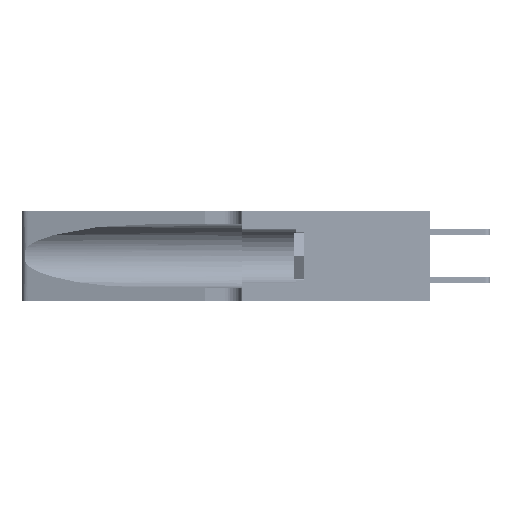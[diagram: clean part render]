
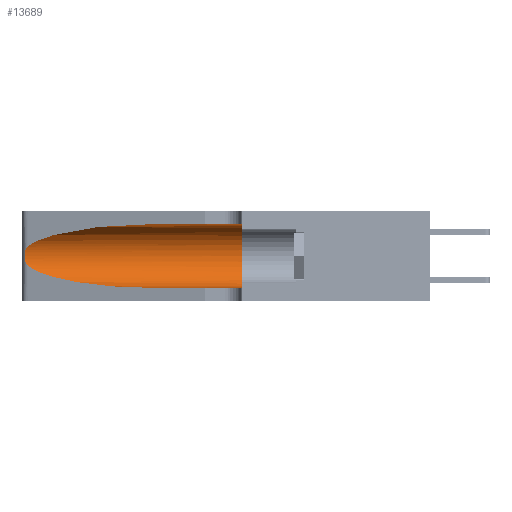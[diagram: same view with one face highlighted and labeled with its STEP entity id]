
A CAD part, left-side view. The second image highlights one B-rep face of the part: STEP entity #13689.
In plain terms, the highlighted cylindrical face has radius 3.308 mm (diameter 6.617 mm), a partial arc.
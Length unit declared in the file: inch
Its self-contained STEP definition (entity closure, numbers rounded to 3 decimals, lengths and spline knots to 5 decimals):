
#970 = CARTESIAN_POINT ( 'NONE',  ( 0.25487, 1.22718, 0.22369 ) ) ;
#1554 = CARTESIAN_POINT ( 'NONE',  ( 0.26075, 1.23896, 0.19203 ) ) ;
#2372 = CARTESIAN_POINT ( 'NONE',  ( 0.25856, 1.23593, 0.16098 ) ) ;
#3456 = CARTESIAN_POINT ( 'NONE',  ( 0.25487, 1.22718, 0.14631 ) ) ;
#3938 = CARTESIAN_POINT ( 'NONE',  ( 0.25487, 1.22718, 0.22369 ) ) ;
#5405 = ORIENTED_EDGE ( 'NONE', *, *, #24044, .T. ) ;
#6078 = EDGE_CURVE ( 'NONE', #14288, #38441, #24843, .T. ) ;
#6222 = EDGE_CURVE ( 'NONE', #24188, #38441, #10200, .T. ) ;
#6293 = VECTOR ( 'NONE', #38115, 39.37008 ) ;
#6353 = ORIENTED_EDGE ( 'NONE', *, *, #6222, .F. ) ;
#7549 = CARTESIAN_POINT ( 'NONE',  ( 0.1305, 0.72297, 0.31525 ) ) ;
#8357 = CARTESIAN_POINT ( 'NONE',  ( 0.1305, 0.35, 0.05475 ) ) ;
#8794 =( BOUNDED_CURVE ( )  B_SPLINE_CURVE ( 3, ( #12885, #34655, #16404, #22267 ),
 .UNSPECIFIED., .F., .F. ) 
 B_SPLINE_CURVE_WITH_KNOTS ( ( 4, 4 ),
 ( 3.44316, 4.71239 ),
 .UNSPECIFIED. ) 
 CURVE ( )  GEOMETRIC_REPRESENTATION_ITEM ( )  RATIONAL_B_SPLINE_CURVE ( ( 1., 0.87, 0.87, 1. ) ) 
 REPRESENTATION_ITEM ( '' )  );
#9586 = FACE_OUTER_BOUND ( 'NONE', #21133, .T. ) ;
#9924 = EDGE_CURVE ( 'NONE', #34025, #24188, #18055, .T. ) ;
#10067 = ORIENTED_EDGE ( 'NONE', *, *, #10087, .T. ) ;
#10087 = EDGE_CURVE ( 'NONE', #34557, #23011, #29959, .T. ) ;
#10200 = CIRCLE ( 'NONE', #36491, 0.13025 ) ;
#11184 = CARTESIAN_POINT ( 'NONE',  ( 0.2373, 1.15595, 0.28018 ) ) ;
#11263 = CARTESIAN_POINT ( 'NONE',  ( 0.25787, 1.23484, 0.2124 ) ) ;
#11590 = CARTESIAN_POINT ( 'NONE',  ( 0.25487, 1.22718, 0.22369 ) ) ;
#12116 = CARTESIAN_POINT ( 'NONE',  ( 0.1305, 0.35, 0.31525 ) ) ;
#12885 = CARTESIAN_POINT ( 'NONE',  ( 0.25487, 1.22718, 0.14631 ) ) ;
#12967 = ORIENTED_EDGE ( 'NONE', *, *, #6078, .T. ) ;
#13513 = CYLINDRICAL_SURFACE ( 'NONE', #17879, 0.13025 ) ;
#13689 = ADVANCED_FACE ( 'NONE', ( #9586 ), #13513, .F. ) ;
#14288 = VERTEX_POINT ( 'NONE', #37192 ) ;
#15039 = CARTESIAN_POINT ( 'NONE',  ( 0.26017, 1.23833, 0.17102 ) ) ;
#15421 = DIRECTION ( 'NONE',  ( 0., -1., 0. ) ) ;
#16009 = EDGE_CURVE ( 'NONE', #23011, #14288, #8794, .T. ) ;
#16404 = CARTESIAN_POINT ( 'NONE',  ( 0.18966, 0.96281, 0.05475 ) ) ;
#16839 = CARTESIAN_POINT ( 'NONE',  ( 0.25555, 1.22994, 0.2215 ) ) ;
#17711 = CARTESIAN_POINT ( 'NONE',  ( 0.18966, 0.96281, 0.31525 ) ) ;
#17795 = CARTESIAN_POINT ( 'NONE',  ( 0.26075, 1.23896, 0.178 ) ) ;
#17811 =( BOUNDED_CURVE ( )  B_SPLINE_CURVE ( 3, ( #36638, #17711, #11184, #11590 ),
 .UNSPECIFIED., .F., .F. ) 
 B_SPLINE_CURVE_WITH_KNOTS ( ( 4, 4 ),
 ( 1.5708, 2.84003 ),
 .UNSPECIFIED. ) 
 CURVE ( )  GEOMETRIC_REPRESENTATION_ITEM ( )  RATIONAL_B_SPLINE_CURVE ( ( 1., 0.87, 0.87, 1. ) ) 
 REPRESENTATION_ITEM ( '' )  );
#17879 = AXIS2_PLACEMENT_3D ( 'NONE', #20970, #15421, #37107 ) ;
#17939 = CARTESIAN_POINT ( 'NONE',  ( 0.25639, 1.23186, 0.15144 ) ) ;
#17942 = DIRECTION ( 'NONE',  ( 0., 1., 0. ) ) ;
#18055 = LINE ( 'NONE', #26381, #20477 ) ;
#18162 = ORIENTED_EDGE ( 'NONE', *, *, #16009, .T. ) ;
#20477 = VECTOR ( 'NONE', #28804, 39.37008 ) ;
#20970 = CARTESIAN_POINT ( 'NONE',  ( 0.1305, 1.61858, 0.185 ) ) ;
#21133 = EDGE_LOOP ( 'NONE', ( #5405, #10067, #18162, #12967, #6353, #23860 ) ) ;
#21653 = CARTESIAN_POINT ( 'NONE',  ( 0.1305, 1.61858, 0.05475 ) ) ;
#21882 = CARTESIAN_POINT ( 'NONE',  ( 0.25639, 1.23184, 0.21858 ) ) ;
#22267 = CARTESIAN_POINT ( 'NONE',  ( 0.1305, 0.72297, 0.05475 ) ) ;
#23011 = VERTEX_POINT ( 'NONE', #3456 ) ;
#23255 = CARTESIAN_POINT ( 'NONE',  ( 0.25854, 1.2359, 0.20912 ) ) ;
#23805 = CARTESIAN_POINT ( 'NONE',  ( 0.25555, 1.22993, 0.14849 ) ) ;
#23860 = ORIENTED_EDGE ( 'NONE', *, *, #9924, .F. ) ;
#24044 = EDGE_CURVE ( 'NONE', #34025, #34557, #17811, .T. ) ;
#24188 = VERTEX_POINT ( 'NONE', #12116 ) ;
#24843 = LINE ( 'NONE', #21653, #6293 ) ;
#26381 = CARTESIAN_POINT ( 'NONE',  ( 0.1305, 1.61858, 0.31525 ) ) ;
#28804 = DIRECTION ( 'NONE',  ( 0., -1., 0. ) ) ;
#29959 = B_SPLINE_CURVE_WITH_KNOTS ( 'NONE', 3,
 ( #970, #16839, #21882, #11263, #23255, #39235, #1554, #17795, #15039, #2372, #36854, #17939, #23805, #33466 ),
 .UNSPECIFIED., .F., .F.,
 ( 4, 2, 2, 2, 2, 2, 4 ),
 ( 0., 0.00027, 0.00053, 0.00107, 0.0016, 0.00187, 0.00214 ),
 .UNSPECIFIED. ) ;
#33466 = CARTESIAN_POINT ( 'NONE',  ( 0.25487, 1.22718, 0.14631 ) ) ;
#33468 = CARTESIAN_POINT ( 'NONE',  ( 0.1305, 0.35, 0.185 ) ) ;
#34025 = VERTEX_POINT ( 'NONE', #7549 ) ;
#34557 = VERTEX_POINT ( 'NONE', #3938 ) ;
#34655 = CARTESIAN_POINT ( 'NONE',  ( 0.2373, 1.15595, 0.08982 ) ) ;
#36491 = AXIS2_PLACEMENT_3D ( 'NONE', #33468, #17942, #39762 ) ;
#36638 = CARTESIAN_POINT ( 'NONE',  ( 0.1305, 0.72297, 0.31525 ) ) ;
#36854 = CARTESIAN_POINT ( 'NONE',  ( 0.25789, 1.23486, 0.15765 ) ) ;
#37107 = DIRECTION ( 'NONE',  ( 0., 0., -1. ) ) ;
#37192 = CARTESIAN_POINT ( 'NONE',  ( 0.1305, 0.72297, 0.05475 ) ) ;
#38115 = DIRECTION ( 'NONE',  ( 0., -1., 0. ) ) ;
#38441 = VERTEX_POINT ( 'NONE', #8357 ) ;
#39235 = CARTESIAN_POINT ( 'NONE',  ( 0.26018, 1.23835, 0.19895 ) ) ;
#39762 = DIRECTION ( 'NONE',  ( 0., 0., 1. ) ) ;
